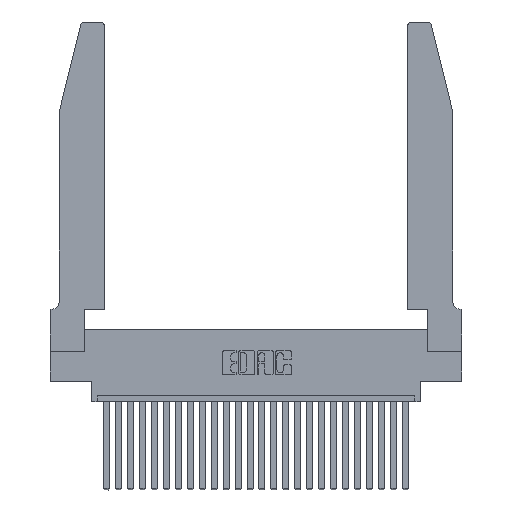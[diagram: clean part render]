
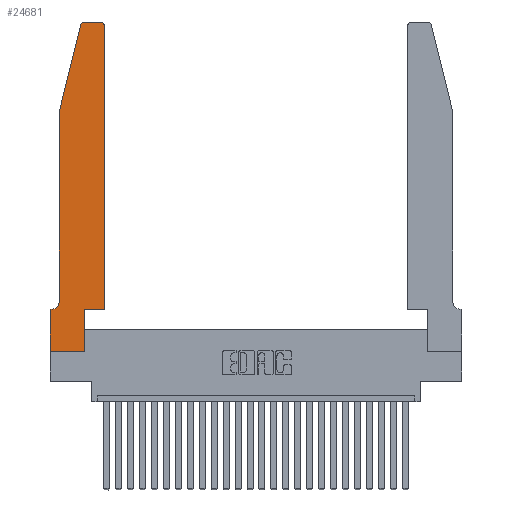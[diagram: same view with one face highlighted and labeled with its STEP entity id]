
A CAD part, top view. The second image highlights one B-rep face of the part: STEP entity #24681.
In plain terms, the highlighted planar face has unit normal (0, 0, 1).
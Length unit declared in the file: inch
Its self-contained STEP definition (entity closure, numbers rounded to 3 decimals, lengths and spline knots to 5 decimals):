
#204 = ORIENTED_EDGE ( 'NONE', *, *, #6631, .T. ) ;
#270 = VERTEX_POINT ( 'NONE', #6247 ) ;
#595 = EDGE_LOOP ( 'NONE', ( #6385, #12979, #9624, #2786, #23445, #204, #17784, #1072, #4424, #22406, #17657, #2718 ) ) ;
#865 = VECTOR ( 'NONE', #7693, 39.37008 ) ;
#1072 = ORIENTED_EDGE ( 'NONE', *, *, #26065, .T. ) ;
#1527 = DIRECTION ( 'NONE',  ( 1., 0., 0. ) ) ;
#1538 = EDGE_CURVE ( 'NONE', #21644, #18651, #18014, .T. ) ;
#1631 = CARTESIAN_POINT ( 'NONE',  ( 0.0055, 0.35, 0.37 ) ) ;
#2414 = EDGE_CURVE ( 'NONE', #20356, #5187, #4210, .T. ) ;
#2469 = VECTOR ( 'NONE', #16918, 39.37008 ) ;
#2718 = ORIENTED_EDGE ( 'NONE', *, *, #21568, .T. ) ;
#2786 = ORIENTED_EDGE ( 'NONE', *, *, #17415, .T. ) ;
#3035 = CARTESIAN_POINT ( 'NONE',  ( 0.0055, 0.42, 0.37 ) ) ;
#3082 = LINE ( 'NONE', #3667, #24129 ) ;
#3667 = CARTESIAN_POINT ( 'NONE',  ( 0.2605, 2.75, 0.37 ) ) ;
#4210 = LINE ( 'NONE', #21960, #11494 ) ;
#4424 = ORIENTED_EDGE ( 'NONE', *, *, #7462, .T. ) ;
#4482 = VERTEX_POINT ( 'NONE', #11020 ) ;
#4651 = CARTESIAN_POINT ( 'NONE',  ( 0.2865, 0.35, 0.37 ) ) ;
#4952 = LINE ( 'NONE', #4651, #20589 ) ;
#5064 = CARTESIAN_POINT ( 'NONE',  ( 0.0755, 2., 0.37 ) ) ;
#5079 = CARTESIAN_POINT ( 'NONE',  ( 0.4505, 0.35, 0.37 ) ) ;
#5128 = FACE_OUTER_BOUND ( 'NONE', #595, .T. ) ;
#5187 = VERTEX_POINT ( 'NONE', #5064 ) ;
#5254 = DIRECTION ( 'NONE',  ( 0., 1., 0. ) ) ;
#5666 = CARTESIAN_POINT ( 'NONE',  ( 0., 0., 0.37 ) ) ;
#5708 = DIRECTION ( 'NONE',  ( 1., 0., 0. ) ) ;
#5895 = DIRECTION ( 'NONE',  ( 0., 0., 1. ) ) ;
#6117 = EDGE_CURVE ( 'NONE', #19243, #24645, #16778, .T. ) ;
#6123 = DIRECTION ( 'NONE',  ( 0., -1., 0. ) ) ;
#6247 = CARTESIAN_POINT ( 'NONE',  ( 0.2865, 0., 0.37 ) ) ;
#6304 = CARTESIAN_POINT ( 'NONE',  ( 0., 0.35, 0.37 ) ) ;
#6368 = CARTESIAN_POINT ( 'NONE',  ( 0.0755, 2., 0.37 ) ) ;
#6385 = ORIENTED_EDGE ( 'NONE', *, *, #17767, .T. ) ;
#6631 = EDGE_CURVE ( 'NONE', #12375, #19243, #14480, .T. ) ;
#6635 = DIRECTION ( 'NONE',  ( 0., 0., 1. ) ) ;
#7432 = VECTOR ( 'NONE', #5254, 39.37008 ) ;
#7462 = EDGE_CURVE ( 'NONE', #270, #7856, #4952, .T. ) ;
#7476 = DIRECTION ( 'NONE',  ( -1., 0., 0. ) ) ;
#7478 = VECTOR ( 'NONE', #7476, 39.37008 ) ;
#7693 = DIRECTION ( 'NONE',  ( 0., -1., 0. ) ) ;
#7856 = VERTEX_POINT ( 'NONE', #16263 ) ;
#7889 = AXIS2_PLACEMENT_3D ( 'NONE', #6304, #6635, #10438 ) ;
#9159 = DIRECTION ( 'NONE',  ( 0., 0., -1. ) ) ;
#9624 = ORIENTED_EDGE ( 'NONE', *, *, #2414, .T. ) ;
#10012 = CIRCLE ( 'NONE', #19574, 0.03 ) ;
#10179 = CARTESIAN_POINT ( 'NONE',  ( 0., 0., 0.37 ) ) ;
#10438 = DIRECTION ( 'NONE',  ( 1., 0., 0. ) ) ;
#11020 = CARTESIAN_POINT ( 'NONE',  ( 0.4205, 2.75, 0.37 ) ) ;
#11054 = LINE ( 'NONE', #17115, #2469 ) ;
#11356 = CARTESIAN_POINT ( 'NONE',  ( 0.4205, 2.72, 0.37 ) ) ;
#11494 = VECTOR ( 'NONE', #17678, 39.37008 ) ;
#11810 = CIRCLE ( 'NONE', #21164, 0.03 ) ;
#11900 = VERTEX_POINT ( 'NONE', #13827 ) ;
#12375 = VERTEX_POINT ( 'NONE', #1631 ) ;
#12979 = ORIENTED_EDGE ( 'NONE', *, *, #19240, .T. ) ;
#13031 = AXIS2_PLACEMENT_3D ( 'NONE', #3035, #9159, #21490 ) ;
#13827 = CARTESIAN_POINT ( 'NONE',  ( 0.0755, 0.42, 0.37 ) ) ;
#14324 = CARTESIAN_POINT ( 'NONE',  ( 0.284, 2.75, 0.37 ) ) ;
#14480 = LINE ( 'NONE', #19697, #7478 ) ;
#15016 = EDGE_CURVE ( 'NONE', #11900, #12375, #22890, .T. ) ;
#15835 = VECTOR ( 'NONE', #6123, 39.37008 ) ;
#16263 = CARTESIAN_POINT ( 'NONE',  ( 0.2865, 0.35, 0.37 ) ) ;
#16455 = PLANE ( 'NONE',  #7889 ) ;
#16778 = LINE ( 'NONE', #5666, #865 ) ;
#16918 = DIRECTION ( 'NONE',  ( 1., 0., 0. ) ) ;
#17115 = CARTESIAN_POINT ( 'NONE',  ( 0., 0., 0.37 ) ) ;
#17372 = DIRECTION ( 'NONE',  ( 1., 0., 0. ) ) ;
#17415 = EDGE_CURVE ( 'NONE', #5187, #11900, #21912, .T. ) ;
#17657 = ORIENTED_EDGE ( 'NONE', *, *, #1538, .T. ) ;
#17678 = DIRECTION ( 'NONE',  ( -0.239, -0.971, 0. ) ) ;
#17767 = EDGE_CURVE ( 'NONE', #4482, #24057, #3082, .T. ) ;
#17784 = ORIENTED_EDGE ( 'NONE', *, *, #6117, .T. ) ;
#17846 = CARTESIAN_POINT ( 'NONE',  ( 0.4505, 0.35, 0.37 ) ) ;
#18014 = LINE ( 'NONE', #21662, #7432 ) ;
#18428 = LINE ( 'NONE', #5079, #25423 ) ;
#18651 = VERTEX_POINT ( 'NONE', #20277 ) ;
#19240 = EDGE_CURVE ( 'NONE', #24057, #20356, #10012, .T. ) ;
#19243 = VERTEX_POINT ( 'NONE', #20160 ) ;
#19574 = AXIS2_PLACEMENT_3D ( 'NONE', #24398, #5895, #5708 ) ;
#19697 = CARTESIAN_POINT ( 'NONE',  ( 0.0755, 0.35, 0.37 ) ) ;
#20160 = CARTESIAN_POINT ( 'NONE',  ( 0., 0.35, 0.37 ) ) ;
#20277 = CARTESIAN_POINT ( 'NONE',  ( 0.4505, 2.72, 0.37 ) ) ;
#20356 = VERTEX_POINT ( 'NONE', #22123 ) ;
#20589 = VECTOR ( 'NONE', #21313, 39.37008 ) ;
#21164 = AXIS2_PLACEMENT_3D ( 'NONE', #11356, #25668, #1527 ) ;
#21313 = DIRECTION ( 'NONE',  ( 0., 1., 0. ) ) ;
#21490 = DIRECTION ( 'NONE',  ( -1., 0., 0. ) ) ;
#21568 = EDGE_CURVE ( 'NONE', #18651, #4482, #11810, .T. ) ;
#21644 = VERTEX_POINT ( 'NONE', #17846 ) ;
#21662 = CARTESIAN_POINT ( 'NONE',  ( 0.4505, 0.35, 0.37 ) ) ;
#21912 = LINE ( 'NONE', #6368, #15835 ) ;
#21960 = CARTESIAN_POINT ( 'NONE',  ( 0.0755, 2., 0.37 ) ) ;
#22123 = CARTESIAN_POINT ( 'NONE',  ( 0.25487, 2.72718, 0.37 ) ) ;
#22406 = ORIENTED_EDGE ( 'NONE', *, *, #26153, .T. ) ;
#22890 = CIRCLE ( 'NONE', #13031, 0.07 ) ;
#23445 = ORIENTED_EDGE ( 'NONE', *, *, #15016, .T. ) ;
#24057 = VERTEX_POINT ( 'NONE', #14324 ) ;
#24129 = VECTOR ( 'NONE', #25950, 39.37008 ) ;
#24398 = CARTESIAN_POINT ( 'NONE',  ( 0.284, 2.72, 0.37 ) ) ;
#24645 = VERTEX_POINT ( 'NONE', #10179 ) ;
#24681 = ADVANCED_FACE ( 'NONE', ( #5128 ), #16455, .T. ) ;
#25423 = VECTOR ( 'NONE', #17372, 39.37008 ) ;
#25668 = DIRECTION ( 'NONE',  ( 0., 0., 1. ) ) ;
#25950 = DIRECTION ( 'NONE',  ( -1., 0., 0. ) ) ;
#26065 = EDGE_CURVE ( 'NONE', #24645, #270, #11054, .T. ) ;
#26153 = EDGE_CURVE ( 'NONE', #7856, #21644, #18428, .T. ) ;
